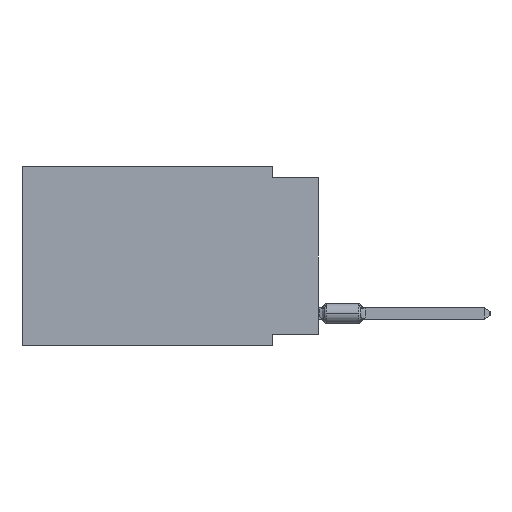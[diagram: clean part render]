
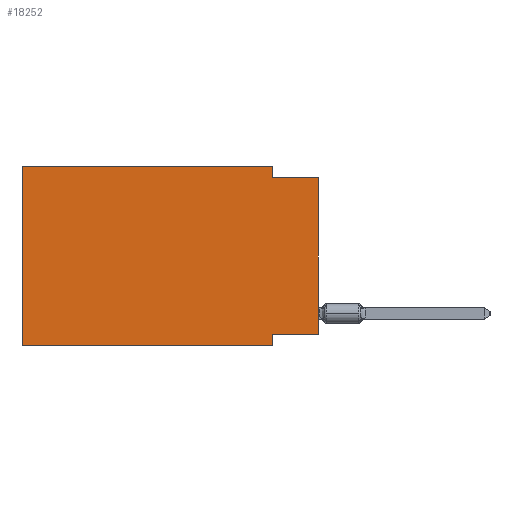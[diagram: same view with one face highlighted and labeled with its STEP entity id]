
A CAD part, left-side view. The second image highlights one B-rep face of the part: STEP entity #18252.
In plain terms, the highlighted planar face has unit normal (-1, 0, 0).
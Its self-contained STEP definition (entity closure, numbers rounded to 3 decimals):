
#528 = ORIENTED_EDGE ( 'NONE', *, *, #31468, .F. ) ;
#1115 = VECTOR ( 'NONE', #42867, 1000. ) ;
#1634 = LINE ( 'NONE', #52505, #8768 ) ;
#3347 = ORIENTED_EDGE ( 'NONE', *, *, #32666, .F. ) ;
#5026 = VERTEX_POINT ( 'NONE', #54760 ) ;
#5927 = EDGE_CURVE ( 'NONE', #33654, #7419, #21669, .T. ) ;
#7388 = FACE_OUTER_BOUND ( 'NONE', #49356, .T. ) ;
#7419 = VERTEX_POINT ( 'NONE', #40706 ) ;
#7992 = CARTESIAN_POINT ( 'NONE',  ( 0., 0., -9.271 ) ) ;
#8545 = DIRECTION ( 'NONE',  ( 0., 1., 0. ) ) ;
#8768 = VECTOR ( 'NONE', #14245, 1000. ) ;
#9116 = VECTOR ( 'NONE', #24706, 1000. ) ;
#9325 = DIRECTION ( 'NONE',  ( 0., -1., 0. ) ) ;
#10768 = CARTESIAN_POINT ( 'NONE',  ( 0., 16.383, 0. ) ) ;
#12268 = CARTESIAN_POINT ( 'NONE',  ( 0., 0., -9.271 ) ) ;
#14065 = ORIENTED_EDGE ( 'NONE', *, *, #29117, .T. ) ;
#14116 = VECTOR ( 'NONE', #9325, 1000. ) ;
#14245 = DIRECTION ( 'NONE',  ( 0., -1., 0. ) ) ;
#14970 = CARTESIAN_POINT ( 'NONE',  ( 0., 2.54, 0. ) ) ;
#15585 = AXIS2_PLACEMENT_3D ( 'NONE', #10768, #15813, #45696 ) ;
#15813 = DIRECTION ( 'NONE',  ( 1., 0., 0. ) ) ;
#17518 = ORIENTED_EDGE ( 'NONE', *, *, #51147, .F. ) ;
#18252 = ADVANCED_FACE ( 'NONE', ( #7388 ), #28393, .F. ) ;
#19057 = CARTESIAN_POINT ( 'NONE',  ( 0., 2.54, -0.635 ) ) ;
#19093 = ORIENTED_EDGE ( 'NONE', *, *, #26755, .F. ) ;
#20952 = VERTEX_POINT ( 'NONE', #12268 ) ;
#21669 = LINE ( 'NONE', #47650, #14116 ) ;
#22106 = VECTOR ( 'NONE', #44591, 1000. ) ;
#22747 = LINE ( 'NONE', #35045, #1115 ) ;
#23336 = LINE ( 'NONE', #23873, #9116 ) ;
#23509 = EDGE_CURVE ( 'NONE', #20952, #43413, #46852, .T. ) ;
#23873 = CARTESIAN_POINT ( 'NONE',  ( 0., 2.54, -9.906 ) ) ;
#24274 = VECTOR ( 'NONE', #41061, 1000. ) ;
#24706 = DIRECTION ( 'NONE',  ( 0., 0., -1. ) ) ;
#24997 = CARTESIAN_POINT ( 'NONE',  ( 0., 0., 0. ) ) ;
#25627 = CARTESIAN_POINT ( 'NONE',  ( 0., 0., -0.635 ) ) ;
#26755 = EDGE_CURVE ( 'NONE', #54352, #34630, #54303, .T. ) ;
#28393 = PLANE ( 'NONE',  #15585 ) ;
#29117 = EDGE_CURVE ( 'NONE', #20952, #36451, #50957, .T. ) ;
#31468 = EDGE_CURVE ( 'NONE', #33654, #5026, #45252, .T. ) ;
#32582 = CARTESIAN_POINT ( 'NONE',  ( 0., 16.383, -9.906 ) ) ;
#32666 = EDGE_CURVE ( 'NONE', #34630, #36451, #22747, .T. ) ;
#33654 = VERTEX_POINT ( 'NONE', #32582 ) ;
#34140 = CARTESIAN_POINT ( 'NONE',  ( 0., 2.54, 0. ) ) ;
#34630 = VERTEX_POINT ( 'NONE', #19057 ) ;
#35045 = CARTESIAN_POINT ( 'NONE',  ( 0., 0., -0.635 ) ) ;
#36451 = VERTEX_POINT ( 'NONE', #25627 ) ;
#40706 = CARTESIAN_POINT ( 'NONE',  ( 0., 2.54, -9.906 ) ) ;
#41061 = DIRECTION ( 'NONE',  ( 0., 0., 1. ) ) ;
#41173 = ORIENTED_EDGE ( 'NONE', *, *, #23509, .F. ) ;
#42867 = DIRECTION ( 'NONE',  ( 0., -1., 0. ) ) ;
#43221 = ORIENTED_EDGE ( 'NONE', *, *, #5927, .T. ) ;
#43413 = VERTEX_POINT ( 'NONE', #46026 ) ;
#44591 = DIRECTION ( 'NONE',  ( 0., 0., -1. ) ) ;
#45252 = LINE ( 'NONE', #53878, #24274 ) ;
#45573 = VECTOR ( 'NONE', #51234, 1000. ) ;
#45696 = DIRECTION ( 'NONE',  ( 0., 0., -1. ) ) ;
#46026 = CARTESIAN_POINT ( 'NONE',  ( 0., 2.54, -9.271 ) ) ;
#46852 = LINE ( 'NONE', #7992, #54556 ) ;
#47650 = CARTESIAN_POINT ( 'NONE',  ( 0., 16.383, -9.906 ) ) ;
#47969 = EDGE_CURVE ( 'NONE', #43413, #7419, #23336, .T. ) ;
#49356 = EDGE_LOOP ( 'NONE', ( #14065, #3347, #19093, #17518, #528, #43221, #54550, #41173 ) ) ;
#50957 = LINE ( 'NONE', #24997, #45573 ) ;
#51147 = EDGE_CURVE ( 'NONE', #5026, #54352, #1634, .T. ) ;
#51234 = DIRECTION ( 'NONE',  ( 0., 0., 1. ) ) ;
#52505 = CARTESIAN_POINT ( 'NONE',  ( 0., 16.383, 0. ) ) ;
#53878 = CARTESIAN_POINT ( 'NONE',  ( 0., 16.383, 0. ) ) ;
#54303 = LINE ( 'NONE', #14970, #22106 ) ;
#54352 = VERTEX_POINT ( 'NONE', #34140 ) ;
#54550 = ORIENTED_EDGE ( 'NONE', *, *, #47969, .F. ) ;
#54556 = VECTOR ( 'NONE', #8545, 1000. ) ;
#54760 = CARTESIAN_POINT ( 'NONE',  ( 0., 16.383, 0. ) ) ;
